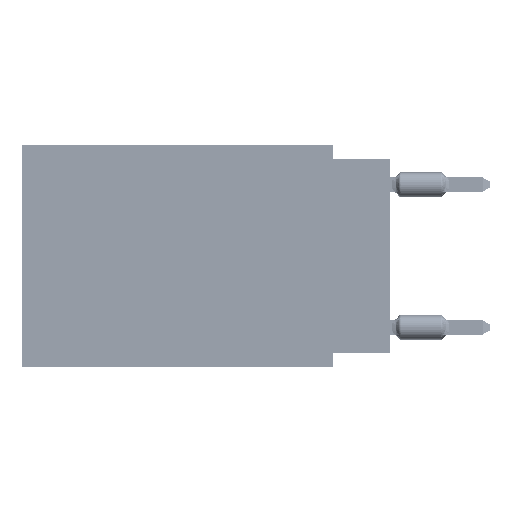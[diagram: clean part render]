
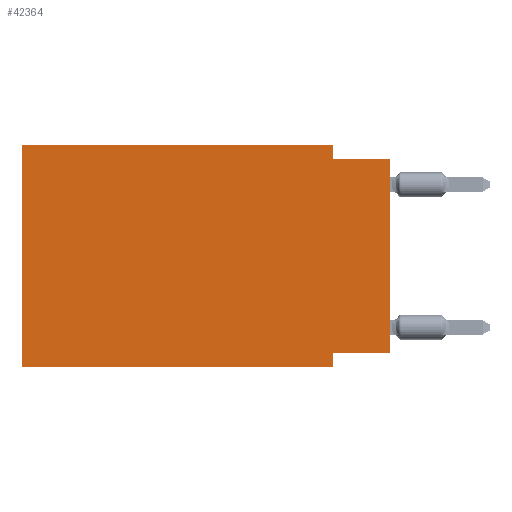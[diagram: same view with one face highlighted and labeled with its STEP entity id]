
A CAD part, left-side view. The second image highlights one B-rep face of the part: STEP entity #42364.
In plain terms, the highlighted planar face has unit normal (-1, 0, 0).
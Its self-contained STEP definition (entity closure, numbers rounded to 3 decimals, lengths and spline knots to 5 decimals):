
#923 = VECTOR ( 'NONE', #76270, 39.37008 ) ;
#1967 = CARTESIAN_POINT ( 'NONE',  ( 0., 0., -0.025 ) ) ;
#2277 = DIRECTION ( 'NONE',  ( 0., 0., -1. ) ) ;
#2327 = VECTOR ( 'NONE', #73898, 39.37008 ) ;
#2900 = VERTEX_POINT ( 'NONE', #4818 ) ;
#3136 = LINE ( 'NONE', #73441, #37218 ) ;
#4185 = CARTESIAN_POINT ( 'NONE',  ( 0., 0., -0.025 ) ) ;
#4818 = CARTESIAN_POINT ( 'NONE',  ( 0., 0.645, -0.39 ) ) ;
#5208 = ORIENTED_EDGE ( 'NONE', *, *, #48710, .F. ) ;
#5577 = LINE ( 'NONE', #77436, #923 ) ;
#5823 = DIRECTION ( 'NONE',  ( 0., 0., 1. ) ) ;
#6425 = EDGE_CURVE ( 'NONE', #56745, #32216, #54504, .T. ) ;
#6857 = CARTESIAN_POINT ( 'NONE',  ( 0., 0.645, 0. ) ) ;
#6996 = FACE_OUTER_BOUND ( 'NONE', #21230, .T. ) ;
#7386 = VECTOR ( 'NONE', #5823, 39.37008 ) ;
#7498 = VECTOR ( 'NONE', #24933, 39.37008 ) ;
#9124 = LINE ( 'NONE', #20131, #2327 ) ;
#9401 = EDGE_CURVE ( 'NONE', #44550, #32216, #75005, .T. ) ;
#11513 = VECTOR ( 'NONE', #50282, 39.37008 ) ;
#11909 = LINE ( 'NONE', #66858, #54653 ) ;
#12483 = VECTOR ( 'NONE', #2277, 39.37008 ) ;
#13064 = ORIENTED_EDGE ( 'NONE', *, *, #9401, .F. ) ;
#20131 = CARTESIAN_POINT ( 'NONE',  ( 0., 0.645, 0. ) ) ;
#20526 = CARTESIAN_POINT ( 'NONE',  ( 0., 0.1, 0. ) ) ;
#21230 = EDGE_LOOP ( 'NONE', ( #38968, #13064, #43387, #5208, #71602, #49633, #40529, #56794 ) ) ;
#21660 = EDGE_CURVE ( 'NONE', #54080, #44550, #11909, .T. ) ;
#24933 = DIRECTION ( 'NONE',  ( 0., -1., 0. ) ) ;
#32216 = VERTEX_POINT ( 'NONE', #4185 ) ;
#37037 = DIRECTION ( 'NONE',  ( 0., 0., -1. ) ) ;
#37218 = VECTOR ( 'NONE', #68707, 39.37008 ) ;
#37251 = DIRECTION ( 'NONE',  ( 1., 0., 0. ) ) ;
#38968 = ORIENTED_EDGE ( 'NONE', *, *, #6425, .T. ) ;
#39121 = VERTEX_POINT ( 'NONE', #45115 ) ;
#39525 = AXIS2_PLACEMENT_3D ( 'NONE', #72585, #37251, #65922 ) ;
#40529 = ORIENTED_EDGE ( 'NONE', *, *, #50545, .F. ) ;
#41580 = CARTESIAN_POINT ( 'NONE',  ( 0., 0., 0. ) ) ;
#42364 = ADVANCED_FACE ( 'NONE', ( #6996 ), #67466, .F. ) ;
#43387 = ORIENTED_EDGE ( 'NONE', *, *, #21660, .F. ) ;
#44198 = CARTESIAN_POINT ( 'NONE',  ( 0., 0., -0.365 ) ) ;
#44550 = VERTEX_POINT ( 'NONE', #73200 ) ;
#44698 = LINE ( 'NONE', #67478, #12483 ) ;
#44992 = VERTEX_POINT ( 'NONE', #68666 ) ;
#45115 = CARTESIAN_POINT ( 'NONE',  ( 0., 0.645, 0. ) ) ;
#45772 = EDGE_CURVE ( 'NONE', #56745, #67898, #5577, .T. ) ;
#48710 = EDGE_CURVE ( 'NONE', #39121, #54080, #60648, .T. ) ;
#49172 = EDGE_CURVE ( 'NONE', #2900, #39121, #9124, .T. ) ;
#49633 = ORIENTED_EDGE ( 'NONE', *, *, #71553, .T. ) ;
#50282 = DIRECTION ( 'NONE',  ( 0., -1., 0. ) ) ;
#50545 = EDGE_CURVE ( 'NONE', #67898, #44992, #44698, .T. ) ;
#54080 = VERTEX_POINT ( 'NONE', #20526 ) ;
#54504 = LINE ( 'NONE', #41580, #7386 ) ;
#54653 = VECTOR ( 'NONE', #37037, 39.37008 ) ;
#56745 = VERTEX_POINT ( 'NONE', #44198 ) ;
#56794 = ORIENTED_EDGE ( 'NONE', *, *, #45772, .F. ) ;
#60648 = LINE ( 'NONE', #6857, #7498 ) ;
#63672 = CARTESIAN_POINT ( 'NONE',  ( 0., 0.1, -0.365 ) ) ;
#65922 = DIRECTION ( 'NONE',  ( 0., 0., -1. ) ) ;
#66858 = CARTESIAN_POINT ( 'NONE',  ( 0., 0.1, 0. ) ) ;
#67466 = PLANE ( 'NONE',  #39525 ) ;
#67478 = CARTESIAN_POINT ( 'NONE',  ( 0., 0.1, -0.39 ) ) ;
#67898 = VERTEX_POINT ( 'NONE', #63672 ) ;
#68666 = CARTESIAN_POINT ( 'NONE',  ( 0., 0.1, -0.39 ) ) ;
#68707 = DIRECTION ( 'NONE',  ( 0., -1., 0. ) ) ;
#71553 = EDGE_CURVE ( 'NONE', #2900, #44992, #3136, .T. ) ;
#71602 = ORIENTED_EDGE ( 'NONE', *, *, #49172, .F. ) ;
#72585 = CARTESIAN_POINT ( 'NONE',  ( 0., 0.645, 0. ) ) ;
#73200 = CARTESIAN_POINT ( 'NONE',  ( 0., 0.1, -0.025 ) ) ;
#73441 = CARTESIAN_POINT ( 'NONE',  ( 0., 0.645, -0.39 ) ) ;
#73898 = DIRECTION ( 'NONE',  ( 0., 0., 1. ) ) ;
#75005 = LINE ( 'NONE', #1967, #11513 ) ;
#76270 = DIRECTION ( 'NONE',  ( 0., 1., 0. ) ) ;
#77436 = CARTESIAN_POINT ( 'NONE',  ( 0., 0., -0.365 ) ) ;
